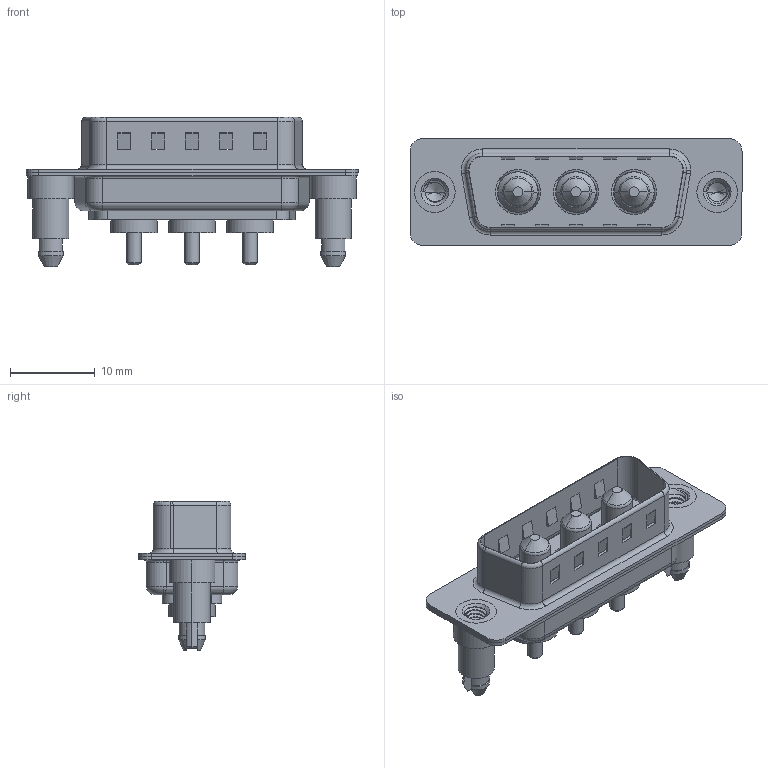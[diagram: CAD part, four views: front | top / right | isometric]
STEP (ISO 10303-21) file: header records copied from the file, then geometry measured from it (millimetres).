
FILE_DESCRIPTION (( 'STEP AP203' ), '1' );
FILE_NAME ('627-3W3-624-1ND.STEP', '2019-05-24T16:53:27', ( '' ), ( '' ), 'SwSTEP 2.0', 'SolidWorks 2016', '' );
FILE_SCHEMA (( 'CONFIG_CONTROL_DESIGN' ));
Length unit declared in the file: millimetre
Products named in the file (7): 627-3W3-624-1ND; 627Combo Housing_3W3; 627Combo Shell Rear_15 Contacts; 627Combo Shell Front_15 Contacts; 627Combo Threaded Boardlock_D; Power Pin_10A S; 627Combo Threaded Boardlock_5
Assembly tree (8 placements, depth 2):
  627-3W3-624-1ND
    627Combo Housing_3W3
    627Combo Shell Rear_15 Contacts
    627Combo Shell Front_15 Contacts
    627Combo Threaded Boardlock_D
    Power Pin_10A S  x3
    627Combo Threaded Boardlock_5
Bounding box: 39.15 x 12.6 x 17.6 mm (x, y, z)
Volume: 2139.7 mm3; surface area: 5005 mm2
Topology: 11 solids, 11 shells, 518 faces, 1264 edges, 792 vertices
Faces by surface type: cylinder 230, plane 185, torus 56, cone 34, bspline 13
Entity records: 17822 total; most frequent: CARTESIAN_POINT 6361, DIRECTION 2268, ORIENTED_EDGE 2224, EDGE_CURVE 1112, AXIS2_PLACEMENT_3D 847, VERTEX_POINT 704, LINE 574, VECTOR 574
